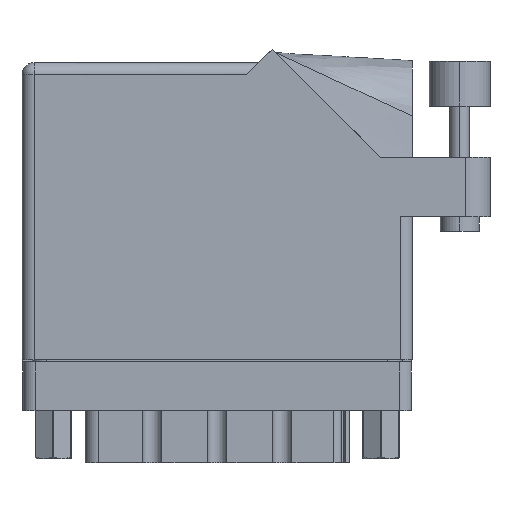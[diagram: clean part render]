
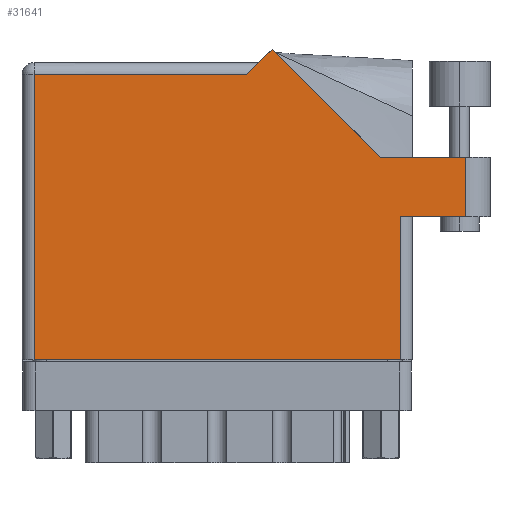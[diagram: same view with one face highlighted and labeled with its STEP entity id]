
A CAD part, front view. The second image highlights one B-rep face of the part: STEP entity #31641.
In plain terms, the highlighted face is planar.
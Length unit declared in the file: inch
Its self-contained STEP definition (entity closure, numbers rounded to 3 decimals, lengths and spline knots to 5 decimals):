
#446 = CARTESIAN_POINT ( 'NONE',  ( 1.948, 0., 0. ) ) ;
#571 = DIRECTION ( 'NONE',  ( 1., 0., 0. ) ) ;
#1127 = CARTESIAN_POINT ( 'NONE',  ( 1.155, 1.468, 0. ) ) ;
#2481 = EDGE_CURVE ( 'NONE', #2942, #28017, #41838, .T. ) ;
#2771 = CARTESIAN_POINT ( 'NONE',  ( 0., 1.468, 0. ) ) ;
#2884 = EDGE_CURVE ( 'NONE', #6635, #32537, #35691, .T. ) ;
#2942 = VERTEX_POINT ( 'NONE', #10337 ) ;
#3224 = FACE_OUTER_BOUND ( 'NONE', #16242, .T. ) ;
#4123 = LINE ( 'NONE', #37701, #40764 ) ;
#6635 = VERTEX_POINT ( 'NONE', #446 ) ;
#7231 = CARTESIAN_POINT ( 'NONE',  ( 0., 0., 0. ) ) ;
#8137 = LINE ( 'NONE', #31795, #18747 ) ;
#8619 = VERTEX_POINT ( 'NONE', #12607 ) ;
#8750 = ORIENTED_EDGE ( 'NONE', *, *, #33082, .T. ) ;
#9501 = VECTOR ( 'NONE', #17426, 39.37008 ) ;
#10337 = CARTESIAN_POINT ( 'NONE',  ( 1.28771, 1.60071, 0. ) ) ;
#10686 = CARTESIAN_POINT ( 'NONE',  ( 2.41, 1.044, 0. ) ) ;
#12607 = CARTESIAN_POINT ( 'NONE',  ( 2.285, 0.737, 0. ) ) ;
#13031 = VERTEX_POINT ( 'NONE', #42163 ) ;
#13265 = ORIENTED_EDGE ( 'NONE', *, *, #18154, .T. ) ;
#13915 = DIRECTION ( 'NONE',  ( -1., 0., 0. ) ) ;
#15820 = PLANE ( 'NONE',  #19446 ) ;
#15972 = DIRECTION ( 'NONE',  ( -1., 0., 0. ) ) ;
#16242 = EDGE_LOOP ( 'NONE', ( #8750, #22693, #37768, #13265, #35989, #41134, #40598, #25384, #35369 ) ) ;
#16494 = CARTESIAN_POINT ( 'NONE',  ( 1.948, 0.737, 0. ) ) ;
#17048 = EDGE_CURVE ( 'NONE', #40019, #6635, #19488, .T. ) ;
#17426 = DIRECTION ( 'NONE',  ( -1., 0., 0. ) ) ;
#17930 = VERTEX_POINT ( 'NONE', #26076 ) ;
#18154 = EDGE_CURVE ( 'NONE', #18266, #2942, #4123, .T. ) ;
#18266 = VERTEX_POINT ( 'NONE', #41573 ) ;
#18747 = VECTOR ( 'NONE', #21262, 39.37008 ) ;
#19446 = AXIS2_PLACEMENT_3D ( 'NONE', #23282, #37265, #15972 ) ;
#19488 = LINE ( 'NONE', #7231, #31139 ) ;
#21256 = CARTESIAN_POINT ( 'NONE',  ( 1.948, 0.737, 0. ) ) ;
#21262 = DIRECTION ( 'NONE',  ( 0., -1., 0. ) ) ;
#21424 = CARTESIAN_POINT ( 'NONE',  ( 1.217, 1.53, 0. ) ) ;
#21688 = CARTESIAN_POINT ( 'NONE',  ( 0.062, 0., 0. ) ) ;
#22693 = ORIENTED_EDGE ( 'NONE', *, *, #34825, .T. ) ;
#23282 = CARTESIAN_POINT ( 'NONE',  ( 0., 1.53, 0. ) ) ;
#25384 = ORIENTED_EDGE ( 'NONE', *, *, #17048, .T. ) ;
#26076 = CARTESIAN_POINT ( 'NONE',  ( 2.285, 1.044, 0. ) ) ;
#26573 = DIRECTION ( 'NONE',  ( 0., 1., 0. ) ) ;
#26809 = VECTOR ( 'NONE', #35534, 39.37008 ) ;
#26877 = CARTESIAN_POINT ( 'NONE',  ( 2.285, 1.044, 0. ) ) ;
#28017 = VERTEX_POINT ( 'NONE', #1127 ) ;
#29009 = LINE ( 'NONE', #26877, #45679 ) ;
#30159 = VECTOR ( 'NONE', #13915, 39.37008 ) ;
#31139 = VECTOR ( 'NONE', #571, 39.37008 ) ;
#31641 = ADVANCED_FACE ( 'NONE', ( #3224 ), #15820, .F. ) ;
#31795 = CARTESIAN_POINT ( 'NONE',  ( 0.062, 0., 0. ) ) ;
#31834 = VECTOR ( 'NONE', #38650, 39.37008 ) ;
#31965 = EDGE_CURVE ( 'NONE', #13031, #40019, #8137, .T. ) ;
#32537 = VERTEX_POINT ( 'NONE', #16494 ) ;
#33082 = EDGE_CURVE ( 'NONE', #32537, #8619, #38074, .T. ) ;
#34077 = EDGE_CURVE ( 'NONE', #28017, #13031, #39657, .T. ) ;
#34825 = EDGE_CURVE ( 'NONE', #8619, #17930, #29009, .T. ) ;
#34904 = EDGE_CURVE ( 'NONE', #17930, #18266, #43457, .T. ) ;
#35369 = ORIENTED_EDGE ( 'NONE', *, *, #2884, .T. ) ;
#35534 = DIRECTION ( 'NONE',  ( 0., 1., 0. ) ) ;
#35691 = LINE ( 'NONE', #21256, #26809 ) ;
#35989 = ORIENTED_EDGE ( 'NONE', *, *, #2481, .T. ) ;
#36645 = CARTESIAN_POINT ( 'NONE',  ( 2.01, 0.737, 0. ) ) ;
#36964 = VECTOR ( 'NONE', #40508, 39.37008 ) ;
#37265 = DIRECTION ( 'NONE',  ( 0., 0., -1. ) ) ;
#37701 = CARTESIAN_POINT ( 'NONE',  ( 1.84442, 1.044, 0. ) ) ;
#37768 = ORIENTED_EDGE ( 'NONE', *, *, #34904, .T. ) ;
#38074 = LINE ( 'NONE', #36645, #36964 ) ;
#38650 = DIRECTION ( 'NONE',  ( -0.707, -0.707, 0. ) ) ;
#39657 = LINE ( 'NONE', #2771, #30159 ) ;
#40019 = VERTEX_POINT ( 'NONE', #21688 ) ;
#40508 = DIRECTION ( 'NONE',  ( 1., 0., 0. ) ) ;
#40598 = ORIENTED_EDGE ( 'NONE', *, *, #31965, .T. ) ;
#40764 = VECTOR ( 'NONE', #45156, 39.37008 ) ;
#41134 = ORIENTED_EDGE ( 'NONE', *, *, #34077, .T. ) ;
#41573 = CARTESIAN_POINT ( 'NONE',  ( 1.84442, 1.044, 0. ) ) ;
#41838 = LINE ( 'NONE', #21424, #31834 ) ;
#42163 = CARTESIAN_POINT ( 'NONE',  ( 0.062, 1.468, 0. ) ) ;
#43457 = LINE ( 'NONE', #10686, #9501 ) ;
#45156 = DIRECTION ( 'NONE',  ( -0.707, 0.707, 0. ) ) ;
#45679 = VECTOR ( 'NONE', #26573, 39.37008 ) ;
